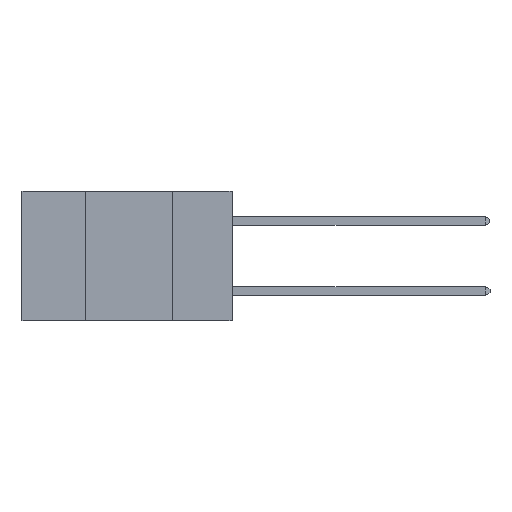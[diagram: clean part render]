
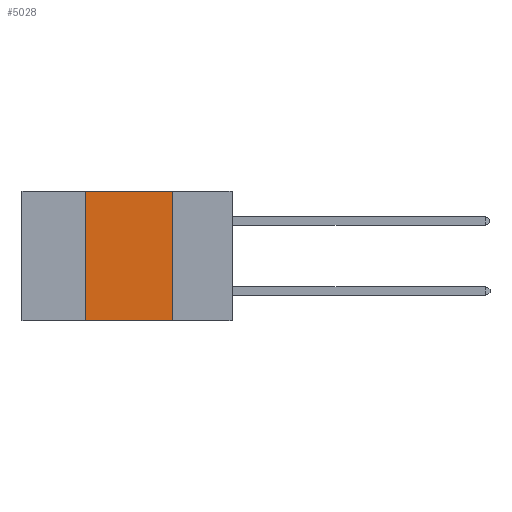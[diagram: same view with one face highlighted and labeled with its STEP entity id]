
A CAD part, left-side view. The second image highlights one B-rep face of the part: STEP entity #5028.
In plain terms, the highlighted planar face has unit normal (-1, 0, 0).
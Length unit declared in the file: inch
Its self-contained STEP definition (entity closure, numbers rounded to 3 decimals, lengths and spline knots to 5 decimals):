
#3 = VECTOR ( 'NONE', #3918, 39.37008 ) ;
#419 = CARTESIAN_POINT ( 'NONE',  ( 0., 0.6, -0.37 ) ) ;
#720 = PLANE ( 'NONE',  #11073 ) ;
#743 = EDGE_CURVE ( 'NONE', #5154, #6359, #4126, .T. ) ;
#1543 = VECTOR ( 'NONE', #6434, 39.37008 ) ;
#1969 = CARTESIAN_POINT ( 'NONE',  ( 0., 0.42, 0. ) ) ;
#2202 = DIRECTION ( 'NONE',  ( 0., 0., -1. ) ) ;
#2291 = EDGE_LOOP ( 'NONE', ( #11705, #8461, #11433, #5232 ) ) ;
#2594 = DIRECTION ( 'NONE',  ( 0., -1., 0. ) ) ;
#2861 = CARTESIAN_POINT ( 'NONE',  ( 0., 0.6, 0. ) ) ;
#3084 = EDGE_CURVE ( 'NONE', #5154, #8512, #10419, .T. ) ;
#3502 = EDGE_CURVE ( 'NONE', #11612, #8512, #5647, .T. ) ;
#3918 = DIRECTION ( 'NONE',  ( 0., -1., 0. ) ) ;
#3952 = FACE_OUTER_BOUND ( 'NONE', #2291, .T. ) ;
#4126 = LINE ( 'NONE', #1969, #1543 ) ;
#4693 = EDGE_CURVE ( 'NONE', #6359, #11612, #5760, .T. ) ;
#5028 = ADVANCED_FACE ( 'NONE', ( #3952 ), #720, .F. ) ;
#5154 = VERTEX_POINT ( 'NONE', #7714 ) ;
#5232 = ORIENTED_EDGE ( 'NONE', *, *, #3084, .T. ) ;
#5647 = LINE ( 'NONE', #9106, #8001 ) ;
#5760 = LINE ( 'NONE', #2861, #3 ) ;
#6359 = VERTEX_POINT ( 'NONE', #9005 ) ;
#6434 = DIRECTION ( 'NONE',  ( 0., 0., 1. ) ) ;
#7087 = CARTESIAN_POINT ( 'NONE',  ( 0., 0.17, 0. ) ) ;
#7714 = CARTESIAN_POINT ( 'NONE',  ( 0., 0.42, -0.37 ) ) ;
#8001 = VECTOR ( 'NONE', #2202, 39.37008 ) ;
#8461 = ORIENTED_EDGE ( 'NONE', *, *, #4693, .F. ) ;
#8512 = VERTEX_POINT ( 'NONE', #10649 ) ;
#9005 = CARTESIAN_POINT ( 'NONE',  ( 0., 0.42, 0. ) ) ;
#9106 = CARTESIAN_POINT ( 'NONE',  ( 0., 0.17, 0. ) ) ;
#10419 = LINE ( 'NONE', #419, #12447 ) ;
#10649 = CARTESIAN_POINT ( 'NONE',  ( 0., 0.17, -0.37 ) ) ;
#11073 = AXIS2_PLACEMENT_3D ( 'NONE', #12003, #11365, #11246 ) ;
#11246 = DIRECTION ( 'NONE',  ( 0., 0., -1. ) ) ;
#11365 = DIRECTION ( 'NONE',  ( 1., 0., 0. ) ) ;
#11433 = ORIENTED_EDGE ( 'NONE', *, *, #743, .F. ) ;
#11612 = VERTEX_POINT ( 'NONE', #7087 ) ;
#11705 = ORIENTED_EDGE ( 'NONE', *, *, #3502, .F. ) ;
#12003 = CARTESIAN_POINT ( 'NONE',  ( 0., 0.6, 0. ) ) ;
#12447 = VECTOR ( 'NONE', #2594, 39.37008 ) ;
